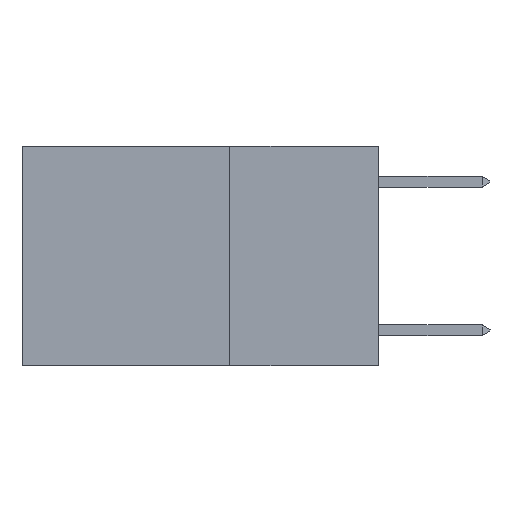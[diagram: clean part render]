
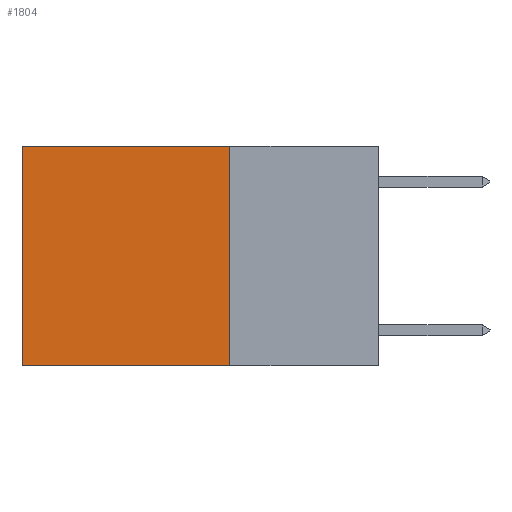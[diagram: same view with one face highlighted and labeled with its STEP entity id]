
A CAD part, left-side view. The second image highlights one B-rep face of the part: STEP entity #1804.
In plain terms, the highlighted planar face has unit normal (-1, 0, 0).
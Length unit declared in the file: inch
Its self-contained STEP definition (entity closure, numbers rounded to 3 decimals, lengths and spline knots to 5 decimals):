
#474 = DIRECTION ( 'NONE',  ( 1., 0., 0. ) ) ;
#1804 = ADVANCED_FACE ( 'NONE', ( #8175 ), #15257, .F. ) ;
#2290 = LINE ( 'NONE', #4951, #7632 ) ;
#2663 = AXIS2_PLACEMENT_3D ( 'NONE', #10966, #474, #15159 ) ;
#3553 = VECTOR ( 'NONE', #5283, 39.37008 ) ;
#4591 = LINE ( 'NONE', #5195, #20878 ) ;
#4787 = VERTEX_POINT ( 'NONE', #14265 ) ;
#4951 = CARTESIAN_POINT ( 'NONE',  ( 0.2625, 0.6, 0. ) ) ;
#5195 = CARTESIAN_POINT ( 'NONE',  ( 0.2625, 0.25, 0. ) ) ;
#5283 = DIRECTION ( 'NONE',  ( 0., 1., 0. ) ) ;
#6230 = LINE ( 'NONE', #26746, #3553 ) ;
#6457 = VERTEX_POINT ( 'NONE', #26794 ) ;
#7632 = VECTOR ( 'NONE', #17754, 39.37008 ) ;
#7906 = EDGE_CURVE ( 'NONE', #4787, #6457, #2290, .T. ) ;
#8164 = EDGE_CURVE ( 'NONE', #27016, #19427, #20264, .T. ) ;
#8175 = FACE_OUTER_BOUND ( 'NONE', #8518, .T. ) ;
#8518 = EDGE_LOOP ( 'NONE', ( #19590, #22484, #25009, #9635 ) ) ;
#9635 = ORIENTED_EDGE ( 'NONE', *, *, #17999, .T. ) ;
#10966 = CARTESIAN_POINT ( 'NONE',  ( 0.2625, 0.25, 0. ) ) ;
#11562 = DIRECTION ( 'NONE',  ( 0., 1., 0. ) ) ;
#12013 = CARTESIAN_POINT ( 'NONE',  ( 0.2625, 0.25, 0. ) ) ;
#14265 = CARTESIAN_POINT ( 'NONE',  ( 0.2625, 0.6, 0. ) ) ;
#14556 = VECTOR ( 'NONE', #22867, 39.37008 ) ;
#15159 = DIRECTION ( 'NONE',  ( 0., 0., -1. ) ) ;
#15257 = PLANE ( 'NONE',  #2663 ) ;
#16072 = CARTESIAN_POINT ( 'NONE',  ( 0.2625, 0.25, 0. ) ) ;
#17754 = DIRECTION ( 'NONE',  ( 0., 0., -1. ) ) ;
#17970 = EDGE_CURVE ( 'NONE', #19427, #6457, #6230, .T. ) ;
#17999 = EDGE_CURVE ( 'NONE', #27016, #4787, #4591, .T. ) ;
#19427 = VERTEX_POINT ( 'NONE', #27234 ) ;
#19590 = ORIENTED_EDGE ( 'NONE', *, *, #7906, .T. ) ;
#20264 = LINE ( 'NONE', #12013, #14556 ) ;
#20878 = VECTOR ( 'NONE', #11562, 39.37008 ) ;
#22484 = ORIENTED_EDGE ( 'NONE', *, *, #17970, .F. ) ;
#22867 = DIRECTION ( 'NONE',  ( 0., 0., -1. ) ) ;
#25009 = ORIENTED_EDGE ( 'NONE', *, *, #8164, .F. ) ;
#26746 = CARTESIAN_POINT ( 'NONE',  ( 0.2625, 0.25, -0.37 ) ) ;
#26794 = CARTESIAN_POINT ( 'NONE',  ( 0.2625, 0.6, -0.37 ) ) ;
#27016 = VERTEX_POINT ( 'NONE', #16072 ) ;
#27234 = CARTESIAN_POINT ( 'NONE',  ( 0.2625, 0.25, -0.37 ) ) ;
